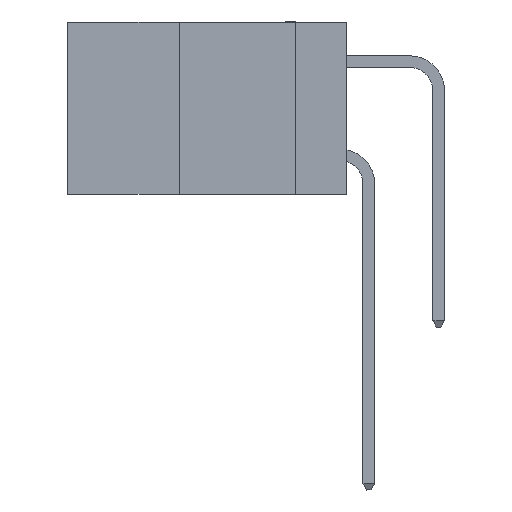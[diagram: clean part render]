
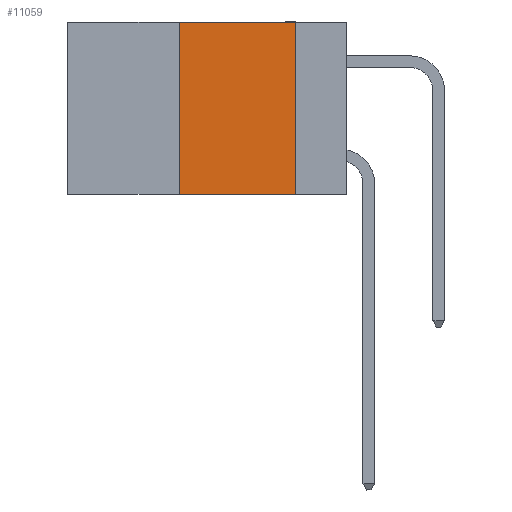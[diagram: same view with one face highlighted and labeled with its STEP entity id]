
A CAD part, left-side view. The second image highlights one B-rep face of the part: STEP entity #11059.
In plain terms, the highlighted planar face has unit normal (-1, 0, 0).
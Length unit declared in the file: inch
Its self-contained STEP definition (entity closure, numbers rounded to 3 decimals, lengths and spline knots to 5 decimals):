
#2453 = CARTESIAN_POINT ( 'NONE',  ( 0., 0.6, -0.37 ) ) ;
#4175 = LINE ( 'NONE', #2453, #16422 ) ;
#5151 = VECTOR ( 'NONE', #28788, 39.37008 ) ;
#6897 = ORIENTED_EDGE ( 'NONE', *, *, #11005, .F. ) ;
#7631 = LINE ( 'NONE', #8171, #12106 ) ;
#8171 = CARTESIAN_POINT ( 'NONE',  ( 0., 0.36, 0. ) ) ;
#8845 = EDGE_LOOP ( 'NONE', ( #13960, #6897, #28279, #24957 ) ) ;
#10019 = DIRECTION ( 'NONE',  ( 0., 0., -1. ) ) ;
#11005 = EDGE_CURVE ( 'NONE', #12969, #13343, #25312, .T. ) ;
#11019 = CARTESIAN_POINT ( 'NONE',  ( 0., 0.36, 0. ) ) ;
#11059 = ADVANCED_FACE ( 'NONE', ( #21967 ), #20602, .F. ) ;
#11230 = EDGE_CURVE ( 'NONE', #12782, #12969, #7631, .T. ) ;
#11686 = CARTESIAN_POINT ( 'NONE',  ( 0., 0.11, 0. ) ) ;
#12106 = VECTOR ( 'NONE', #13440, 39.37008 ) ;
#12782 = VERTEX_POINT ( 'NONE', #32526 ) ;
#12969 = VERTEX_POINT ( 'NONE', #11019 ) ;
#13152 = EDGE_CURVE ( 'NONE', #12782, #29480, #4175, .T. ) ;
#13290 = LINE ( 'NONE', #11686, #5151 ) ;
#13343 = VERTEX_POINT ( 'NONE', #26098 ) ;
#13440 = DIRECTION ( 'NONE',  ( 0., 0., 1. ) ) ;
#13721 = DIRECTION ( 'NONE',  ( 0., -1., 0. ) ) ;
#13952 = AXIS2_PLACEMENT_3D ( 'NONE', #25764, #31175, #10019 ) ;
#13960 = ORIENTED_EDGE ( 'NONE', *, *, #20267, .F. ) ;
#15237 = CARTESIAN_POINT ( 'NONE',  ( 0., 0.11, -0.37 ) ) ;
#16422 = VECTOR ( 'NONE', #13721, 39.37008 ) ;
#18351 = VECTOR ( 'NONE', #27636, 39.37008 ) ;
#19494 = CARTESIAN_POINT ( 'NONE',  ( 0., 0.6, 0. ) ) ;
#20267 = EDGE_CURVE ( 'NONE', #13343, #29480, #13290, .T. ) ;
#20602 = PLANE ( 'NONE',  #13952 ) ;
#21967 = FACE_OUTER_BOUND ( 'NONE', #8845, .T. ) ;
#24957 = ORIENTED_EDGE ( 'NONE', *, *, #13152, .T. ) ;
#25312 = LINE ( 'NONE', #19494, #18351 ) ;
#25764 = CARTESIAN_POINT ( 'NONE',  ( 0., 0.6, 0. ) ) ;
#26098 = CARTESIAN_POINT ( 'NONE',  ( 0., 0.11, 0. ) ) ;
#27636 = DIRECTION ( 'NONE',  ( 0., -1., 0. ) ) ;
#28279 = ORIENTED_EDGE ( 'NONE', *, *, #11230, .F. ) ;
#28788 = DIRECTION ( 'NONE',  ( 0., 0., -1. ) ) ;
#29480 = VERTEX_POINT ( 'NONE', #15237 ) ;
#31175 = DIRECTION ( 'NONE',  ( 1., 0., 0. ) ) ;
#32526 = CARTESIAN_POINT ( 'NONE',  ( 0., 0.36, -0.37 ) ) ;
